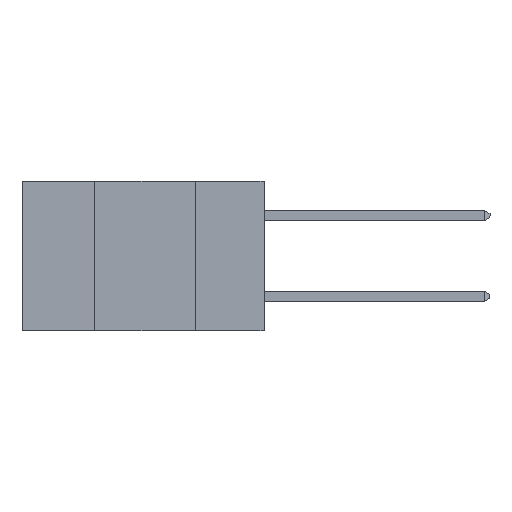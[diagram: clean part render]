
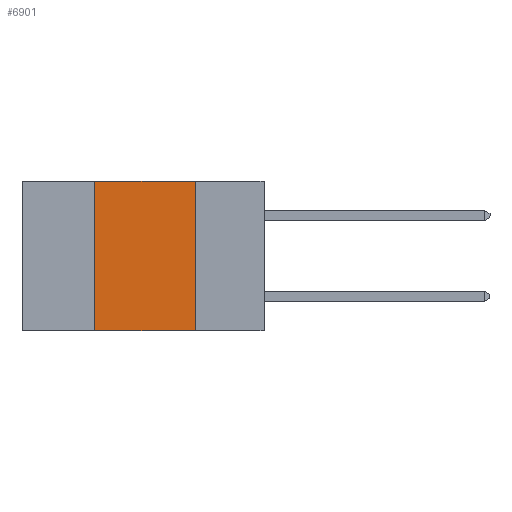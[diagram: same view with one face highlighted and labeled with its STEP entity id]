
A CAD part, left-side view. The second image highlights one B-rep face of the part: STEP entity #6901.
In plain terms, the highlighted planar face has unit normal (-1, 0, 0).
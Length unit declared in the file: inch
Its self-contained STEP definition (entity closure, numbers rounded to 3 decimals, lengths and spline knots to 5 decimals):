
#279 = CARTESIAN_POINT ( 'NONE',  ( 0., 0.17, -0.37 ) ) ;
#282 = ORIENTED_EDGE ( 'NONE', *, *, #4011, .F. ) ;
#442 = VECTOR ( 'NONE', #2643, 39.37008 ) ;
#923 = LINE ( 'NONE', #279, #9572 ) ;
#986 = CARTESIAN_POINT ( 'NONE',  ( 0., 0.6, 0. ) ) ;
#1397 = CARTESIAN_POINT ( 'NONE',  ( 0., 0.42, -0.37 ) ) ;
#1759 = DIRECTION ( 'NONE',  ( 0., 0., -1. ) ) ;
#1974 = DIRECTION ( 'NONE',  ( 0., 0., -1. ) ) ;
#2643 = DIRECTION ( 'NONE',  ( 0., -1., 0. ) ) ;
#2735 = PLANE ( 'NONE',  #3122 ) ;
#2917 = ORIENTED_EDGE ( 'NONE', *, *, #8936, .F. ) ;
#2995 = VERTEX_POINT ( 'NONE', #6842 ) ;
#3122 = AXIS2_PLACEMENT_3D ( 'NONE', #8775, #8722, #1974 ) ;
#3162 = CARTESIAN_POINT ( 'NONE',  ( 0., 0.42, -0.37 ) ) ;
#4011 = EDGE_CURVE ( 'NONE', #7667, #6441, #6339, .T. ) ;
#4035 = DIRECTION ( 'NONE',  ( 0., -1., 0. ) ) ;
#4493 = CARTESIAN_POINT ( 'NONE',  ( 0., 0.42, 0. ) ) ;
#4847 = VECTOR ( 'NONE', #9333, 39.37008 ) ;
#5244 = CARTESIAN_POINT ( 'NONE',  ( 0., 0.17, 0. ) ) ;
#5282 = ORIENTED_EDGE ( 'NONE', *, *, #6655, .F. ) ;
#5550 = CARTESIAN_POINT ( 'NONE',  ( 0., 0.6, -0.37 ) ) ;
#6339 = LINE ( 'NONE', #3162, #4847 ) ;
#6441 = VERTEX_POINT ( 'NONE', #4493 ) ;
#6655 = EDGE_CURVE ( 'NONE', #6441, #8771, #7064, .T. ) ;
#6842 = CARTESIAN_POINT ( 'NONE',  ( 0., 0.17, -0.37 ) ) ;
#6901 = ADVANCED_FACE ( 'NONE', ( #9644 ), #2735, .F. ) ;
#7064 = LINE ( 'NONE', #986, #7359 ) ;
#7359 = VECTOR ( 'NONE', #4035, 39.37008 ) ;
#7667 = VERTEX_POINT ( 'NONE', #1397 ) ;
#8120 = EDGE_CURVE ( 'NONE', #7667, #2995, #9363, .T. ) ;
#8688 = EDGE_LOOP ( 'NONE', ( #2917, #5282, #282, #9337 ) ) ;
#8722 = DIRECTION ( 'NONE',  ( 1., 0., 0. ) ) ;
#8771 = VERTEX_POINT ( 'NONE', #5244 ) ;
#8775 = CARTESIAN_POINT ( 'NONE',  ( 0., 0.6, 0. ) ) ;
#8936 = EDGE_CURVE ( 'NONE', #8771, #2995, #923, .T. ) ;
#9333 = DIRECTION ( 'NONE',  ( 0., 0., 1. ) ) ;
#9337 = ORIENTED_EDGE ( 'NONE', *, *, #8120, .T. ) ;
#9363 = LINE ( 'NONE', #5550, #442 ) ;
#9572 = VECTOR ( 'NONE', #1759, 39.37008 ) ;
#9644 = FACE_OUTER_BOUND ( 'NONE', #8688, .T. ) ;
